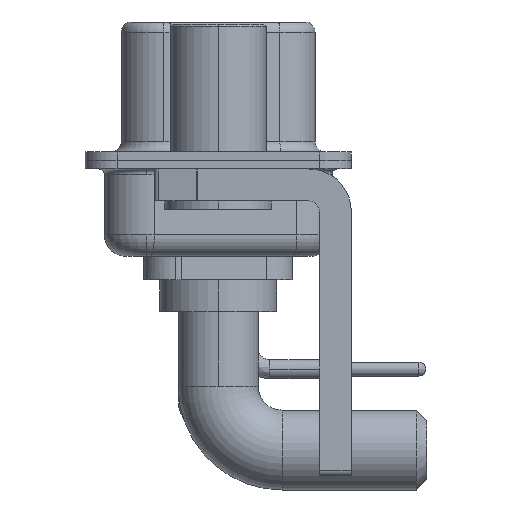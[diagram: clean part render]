
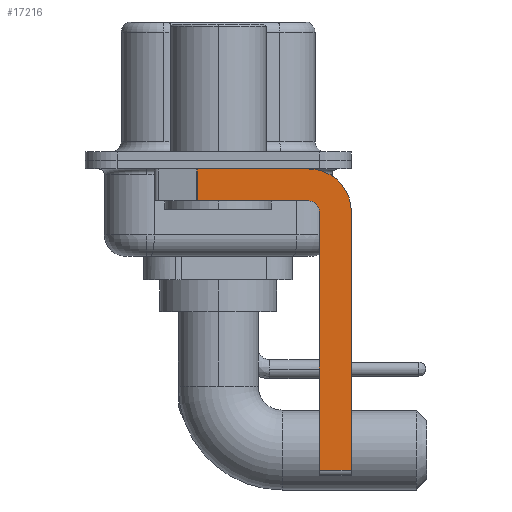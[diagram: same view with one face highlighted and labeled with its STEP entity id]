
A CAD part, left-side view. The second image highlights one B-rep face of the part: STEP entity #17216.
In plain terms, the highlighted planar face has unit normal (-1, 0, 0).
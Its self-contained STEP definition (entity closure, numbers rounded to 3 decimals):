
#446 = LINE ( 'NONE', #6255, #21897 ) ;
#693 = EDGE_CURVE ( 'NONE', #20257, #12840, #9693, .T. ) ;
#894 = CARTESIAN_POINT ( 'NONE',  ( -2.9, -4.25, -0.4 ) ) ;
#1319 = CARTESIAN_POINT ( 'NONE',  ( -2.9, 0.978, -1.9 ) ) ;
#1740 = CARTESIAN_POINT ( 'NONE',  ( -2.9, -4.25, -1.9 ) ) ;
#1778 = CARTESIAN_POINT ( 'NONE',  ( -2.9, -4.25, -1.9 ) ) ;
#2018 = CARTESIAN_POINT ( 'NONE',  ( -2.9, -6.25, -2.4 ) ) ;
#2313 = ORIENTED_EDGE ( 'NONE', *, *, #18391, .T. ) ;
#2340 = DIRECTION ( 'NONE',  ( 0., 0., -1. ) ) ;
#3084 = LINE ( 'NONE', #1319, #12176 ) ;
#4076 = AXIS2_PLACEMENT_3D ( 'NONE', #22942, #17535, #7908 ) ;
#5612 = CARTESIAN_POINT ( 'NONE',  ( -2.9, -4.25, -2.4 ) ) ;
#5744 = DIRECTION ( 'NONE',  ( 0., 0., -1. ) ) ;
#5909 = CARTESIAN_POINT ( 'NONE',  ( -2.9, 3., -0.4 ) ) ;
#6053 = CARTESIAN_POINT ( 'NONE',  ( -2.9, 0.978, -1.9 ) ) ;
#6193 = EDGE_CURVE ( 'NONE', #8952, #12303, #20269, .T. ) ;
#6255 = CARTESIAN_POINT ( 'NONE',  ( -2.9, -6.25, -2.4 ) ) ;
#6287 = LINE ( 'NONE', #5909, #20933 ) ;
#6467 = AXIS2_PLACEMENT_3D ( 'NONE', #19022, #17143, #23174 ) ;
#7149 = CARTESIAN_POINT ( 'NONE',  ( -2.9, -6.25, -14.55 ) ) ;
#7431 = DIRECTION ( 'NONE',  ( 0., 1., 0. ) ) ;
#7632 = EDGE_CURVE ( 'NONE', #13604, #16402, #6287, .T. ) ;
#7908 = DIRECTION ( 'NONE',  ( 0., 0., -1. ) ) ;
#8034 = EDGE_CURVE ( 'NONE', #11655, #12303, #446, .T. ) ;
#8952 = VERTEX_POINT ( 'NONE', #17619 ) ;
#9157 = EDGE_LOOP ( 'NONE', ( #13525, #2313, #19503, #20592, #14455, #17974, #23538, #14804 ) ) ;
#9693 = CIRCLE ( 'NONE', #6467, 0.5 ) ;
#9799 = FACE_OUTER_BOUND ( 'NONE', #9157, .T. ) ;
#10566 = CARTESIAN_POINT ( 'NONE',  ( -2.9, 0.978, -0.4 ) ) ;
#10693 = EDGE_CURVE ( 'NONE', #12840, #12922, #19047, .T. ) ;
#11655 = VERTEX_POINT ( 'NONE', #2018 ) ;
#12176 = VECTOR ( 'NONE', #24418, 1000. ) ;
#12303 = VERTEX_POINT ( 'NONE', #7149 ) ;
#12454 = EDGE_CURVE ( 'NONE', #16402, #11655, #18085, .T. ) ;
#12609 = VECTOR ( 'NONE', #17900, 1000. ) ;
#12840 = VERTEX_POINT ( 'NONE', #1778 ) ;
#12922 = VERTEX_POINT ( 'NONE', #6053 ) ;
#13525 = ORIENTED_EDGE ( 'NONE', *, *, #7632, .F. ) ;
#13604 = VERTEX_POINT ( 'NONE', #10566 ) ;
#14455 = ORIENTED_EDGE ( 'NONE', *, *, #20145, .F. ) ;
#14804 = ORIENTED_EDGE ( 'NONE', *, *, #12454, .F. ) ;
#15250 = PLANE ( 'NONE',  #4076 ) ;
#16402 = VERTEX_POINT ( 'NONE', #894 ) ;
#17143 = DIRECTION ( 'NONE',  ( -1., 0., 0. ) ) ;
#17216 = ADVANCED_FACE ( 'NONE', ( #9799 ), #15250, .F. ) ;
#17535 = DIRECTION ( 'NONE',  ( 1., 0., 0. ) ) ;
#17619 = CARTESIAN_POINT ( 'NONE',  ( -2.9, -4.75, -14.55 ) ) ;
#17900 = DIRECTION ( 'NONE',  ( 0., 0., 1. ) ) ;
#17974 = ORIENTED_EDGE ( 'NONE', *, *, #6193, .T. ) ;
#18085 = CIRCLE ( 'NONE', #24914, 2. ) ;
#18135 = DIRECTION ( 'NONE',  ( 0., -1., 0. ) ) ;
#18391 = EDGE_CURVE ( 'NONE', #13604, #12922, #3084, .T. ) ;
#19022 = CARTESIAN_POINT ( 'NONE',  ( -2.9, -4.25, -2.4 ) ) ;
#19047 = LINE ( 'NONE', #1740, #21620 ) ;
#19259 = DIRECTION ( 'NONE',  ( 1., 0., 0. ) ) ;
#19281 = CARTESIAN_POINT ( 'NONE',  ( -2.9, -4.75, -14.8 ) ) ;
#19408 = LINE ( 'NONE', #19281, #12609 ) ;
#19503 = ORIENTED_EDGE ( 'NONE', *, *, #10693, .F. ) ;
#20145 = EDGE_CURVE ( 'NONE', #8952, #20257, #19408, .T. ) ;
#20257 = VERTEX_POINT ( 'NONE', #23801 ) ;
#20269 = LINE ( 'NONE', #22534, #22895 ) ;
#20592 = ORIENTED_EDGE ( 'NONE', *, *, #693, .F. ) ;
#20933 = VECTOR ( 'NONE', #21688, 1000. ) ;
#21620 = VECTOR ( 'NONE', #7431, 1000. ) ;
#21688 = DIRECTION ( 'NONE',  ( 0., -1., 0. ) ) ;
#21897 = VECTOR ( 'NONE', #2340, 1000. ) ;
#22534 = CARTESIAN_POINT ( 'NONE',  ( -2.9, -4.25, -14.55 ) ) ;
#22895 = VECTOR ( 'NONE', #18135, 1000. ) ;
#22942 = CARTESIAN_POINT ( 'NONE',  ( -2.9, -4.25, -2.4 ) ) ;
#23174 = DIRECTION ( 'NONE',  ( 0., 0., 1. ) ) ;
#23538 = ORIENTED_EDGE ( 'NONE', *, *, #8034, .F. ) ;
#23801 = CARTESIAN_POINT ( 'NONE',  ( -2.9, -4.75, -2.4 ) ) ;
#24418 = DIRECTION ( 'NONE',  ( 0., 0., -1. ) ) ;
#24914 = AXIS2_PLACEMENT_3D ( 'NONE', #5612, #19259, #5744 ) ;
